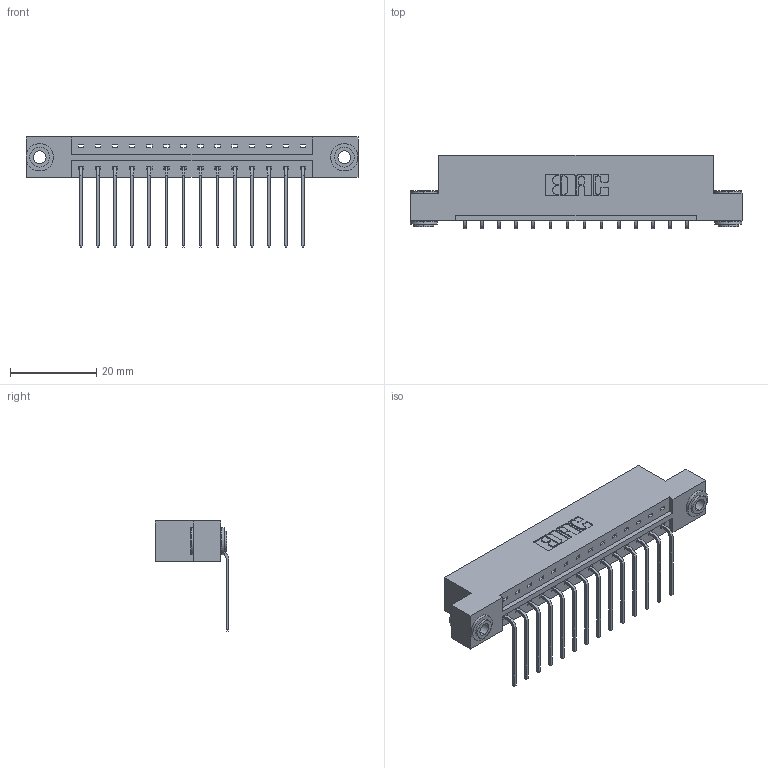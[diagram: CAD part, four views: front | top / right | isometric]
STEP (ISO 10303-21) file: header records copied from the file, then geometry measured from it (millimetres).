
FILE_DESCRIPTION (( 'STEP AP203' ), '1' );
FILE_NAME ('333-014-559-103.STEP', '2018-08-01T03:11:37', ( '' ), ( '' ), 'SwSTEP 2.0', 'SolidWorks 2016', '' );
FILE_SCHEMA (( 'CONFIG_CONTROL_DESIGN' ));
Length unit declared in the file: inch
Products named in the file (4): 345-292-001_558 559 Tail - 1; 345-250-002_345-250-002-102; 333-014-559-103; 333 Part_Flush - .156 Dia - TH
Assembly tree (17 placements, depth 2):
  333-014-559-103
    333 Part_Flush - .156 Dia - TH
    345-292-001_558 559 Tail - 1  x14
    345-250-002_345-250-002-102  x2
Bounding box: 77.01 x 17.09 x 25.53 mm (x, y, z)
Volume: 7574.9 mm3; surface area: 8526.2 mm2
Topology: 17 solids, 17 shells, 992 faces, 2935 edges, 1934 vertices
Faces by surface type: plane 696, cylinder 288, cone 8
Entity records: 12914 total; most frequent: CARTESIAN_POINT 2211, ORIENTED_EDGE 2154, DIRECTION 1955, EDGE_CURVE 1077, VECTOR 925, LINE 925, VERTEX_POINT 714, AXIS2_PLACEMENT_3D 515
